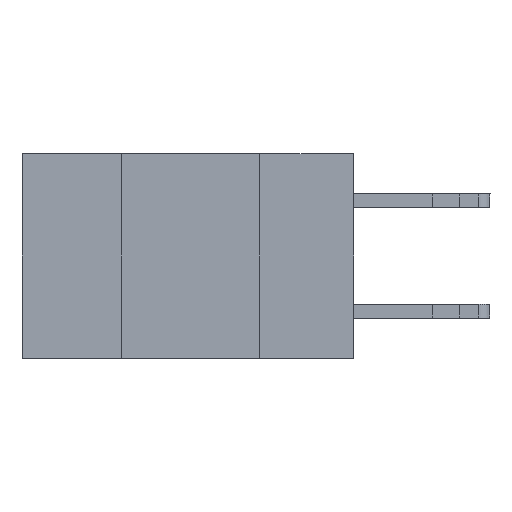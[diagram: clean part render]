
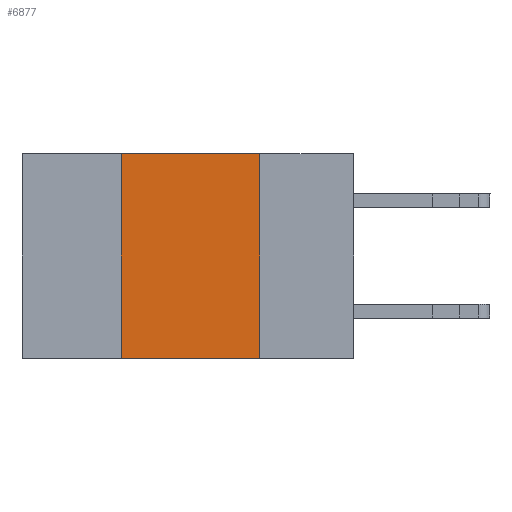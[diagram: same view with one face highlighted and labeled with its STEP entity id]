
A CAD part, left-side view. The second image highlights one B-rep face of the part: STEP entity #6877.
In plain terms, the highlighted planar face has unit normal (-1, 0, 0).
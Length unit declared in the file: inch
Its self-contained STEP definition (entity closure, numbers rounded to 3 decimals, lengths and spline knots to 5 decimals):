
#1101 = EDGE_CURVE ( 'NONE', #8065, #19964, #21507, .T. ) ;
#2244 = VECTOR ( 'NONE', #11091, 39.37008 ) ;
#2430 = PLANE ( 'NONE',  #13009 ) ;
#3468 = CARTESIAN_POINT ( 'NONE',  ( 0., 0.42, 0. ) ) ;
#4694 = VERTEX_POINT ( 'NONE', #5592 ) ;
#5592 = CARTESIAN_POINT ( 'NONE',  ( 0., 0.17, 0. ) ) ;
#5796 = CARTESIAN_POINT ( 'NONE',  ( 0., 0.17, 0. ) ) ;
#6453 = ORIENTED_EDGE ( 'NONE', *, *, #11151, .F. ) ;
#6877 = ADVANCED_FACE ( 'NONE', ( #11033 ), #2430, .F. ) ;
#7708 = LINE ( 'NONE', #5796, #13944 ) ;
#8065 = VERTEX_POINT ( 'NONE', #13789 ) ;
#9285 = LINE ( 'NONE', #12801, #2244 ) ;
#9326 = CARTESIAN_POINT ( 'NONE',  ( 0., 0.6, 0. ) ) ;
#10568 = VECTOR ( 'NONE', #21283, 39.37008 ) ;
#10757 = ORIENTED_EDGE ( 'NONE', *, *, #20185, .F. ) ;
#11033 = FACE_OUTER_BOUND ( 'NONE', #16751, .T. ) ;
#11091 = DIRECTION ( 'NONE',  ( 0., -1., 0. ) ) ;
#11151 = EDGE_CURVE ( 'NONE', #8065, #21552, #19025, .T. ) ;
#12245 = ORIENTED_EDGE ( 'NONE', *, *, #1101, .T. ) ;
#12529 = ORIENTED_EDGE ( 'NONE', *, *, #14180, .F. ) ;
#12801 = CARTESIAN_POINT ( 'NONE',  ( 0., 0.6, 0. ) ) ;
#13009 = AXIS2_PLACEMENT_3D ( 'NONE', #9326, #21482, #15250 ) ;
#13167 = CARTESIAN_POINT ( 'NONE',  ( 0., 0.17, -0.37 ) ) ;
#13789 = CARTESIAN_POINT ( 'NONE',  ( 0., 0.42, -0.37 ) ) ;
#13944 = VECTOR ( 'NONE', #21100, 39.37008 ) ;
#14004 = DIRECTION ( 'NONE',  ( 0., 0., 1. ) ) ;
#14180 = EDGE_CURVE ( 'NONE', #4694, #19964, #7708, .T. ) ;
#15250 = DIRECTION ( 'NONE',  ( 0., 0., -1. ) ) ;
#16010 = VECTOR ( 'NONE', #14004, 39.37008 ) ;
#16751 = EDGE_LOOP ( 'NONE', ( #12529, #10757, #6453, #12245 ) ) ;
#17800 = CARTESIAN_POINT ( 'NONE',  ( 0., 0.42, 0. ) ) ;
#19025 = LINE ( 'NONE', #3468, #16010 ) ;
#19964 = VERTEX_POINT ( 'NONE', #13167 ) ;
#20185 = EDGE_CURVE ( 'NONE', #21552, #4694, #9285, .T. ) ;
#21100 = DIRECTION ( 'NONE',  ( 0., 0., -1. ) ) ;
#21283 = DIRECTION ( 'NONE',  ( 0., -1., 0. ) ) ;
#21390 = CARTESIAN_POINT ( 'NONE',  ( 0., 0.6, -0.37 ) ) ;
#21482 = DIRECTION ( 'NONE',  ( 1., 0., 0. ) ) ;
#21507 = LINE ( 'NONE', #21390, #10568 ) ;
#21552 = VERTEX_POINT ( 'NONE', #17800 ) ;
